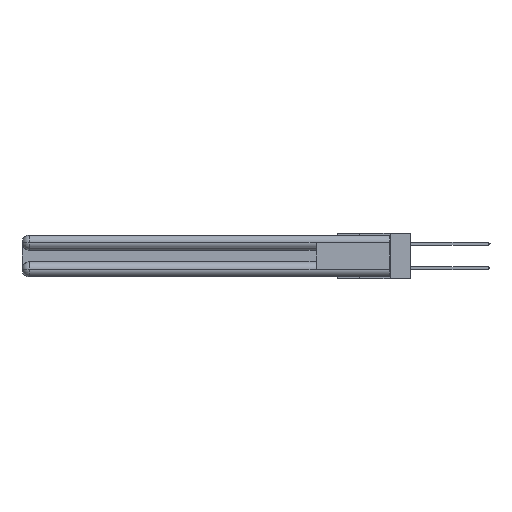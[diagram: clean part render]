
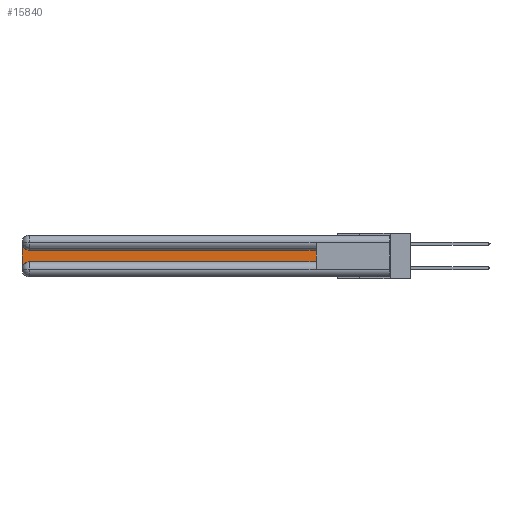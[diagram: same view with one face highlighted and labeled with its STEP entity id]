
A CAD part, left-side view. The second image highlights one B-rep face of the part: STEP entity #15840.
In plain terms, the highlighted planar face has unit normal (-1, 0, 0).
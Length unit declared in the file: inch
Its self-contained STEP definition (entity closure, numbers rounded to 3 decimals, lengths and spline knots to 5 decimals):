
#401 = VERTEX_POINT ( 'NONE', #23673 ) ;
#842 = DIRECTION ( 'NONE',  ( 0., -1., 0. ) ) ;
#939 = VERTEX_POINT ( 'NONE', #5828 ) ;
#1299 = CARTESIAN_POINT ( 'NONE',  ( 0.075, 0.6, -0.2175 ) ) ;
#1949 = EDGE_CURVE ( 'NONE', #9593, #939, #20219, .T. ) ;
#2138 = CARTESIAN_POINT ( 'NONE',  ( 0.075, 3., -0.2775 ) ) ;
#4886 = ORIENTED_EDGE ( 'NONE', *, *, #18905, .T. ) ;
#5600 = DIRECTION ( 'NONE',  ( 0., 1., 0. ) ) ;
#5828 = CARTESIAN_POINT ( 'NONE',  ( 0.075, 2.94, -0.2175 ) ) ;
#6166 = EDGE_LOOP ( 'NONE', ( #17412, #31448, #7244, #15046, #4886, #8875 ) ) ;
#6314 = VECTOR ( 'NONE', #21646, 39.37008 ) ;
#7009 = VECTOR ( 'NONE', #30650, 39.37008 ) ;
#7244 = ORIENTED_EDGE ( 'NONE', *, *, #7268, .T. ) ;
#7268 = EDGE_CURVE ( 'NONE', #401, #9593, #13897, .T. ) ;
#8222 = CARTESIAN_POINT ( 'NONE',  ( 0.075, 3., -0.1225 ) ) ;
#8849 = LINE ( 'NONE', #20236, #29769 ) ;
#8875 = ORIENTED_EDGE ( 'NONE', *, *, #17406, .T. ) ;
#9230 = VECTOR ( 'NONE', #842, 39.37008 ) ;
#9508 = DIRECTION ( 'NONE',  ( 0., 0., -1. ) ) ;
#9593 = VERTEX_POINT ( 'NONE', #2138 ) ;
#9915 = EDGE_CURVE ( 'NONE', #18895, #13813, #8849, .T. ) ;
#12706 = CARTESIAN_POINT ( 'NONE',  ( 0.075, 0.6, -0.2175 ) ) ;
#13439 = LINE ( 'NONE', #1299, #7009 ) ;
#13813 = VERTEX_POINT ( 'NONE', #14164 ) ;
#13897 = LINE ( 'NONE', #16421, #6314 ) ;
#14044 = CARTESIAN_POINT ( 'NONE',  ( 0.075, 0.6, -0.2175 ) ) ;
#14164 = CARTESIAN_POINT ( 'NONE',  ( 0.075, 2.94, -0.1225 ) ) ;
#15046 = ORIENTED_EDGE ( 'NONE', *, *, #1949, .T. ) ;
#15840 = ADVANCED_FACE ( 'NONE', ( #29545 ), #22667, .F. ) ;
#16421 = CARTESIAN_POINT ( 'NONE',  ( 0.075, 3., -0.2175 ) ) ;
#17406 = EDGE_CURVE ( 'NONE', #29827, #18895, #13439, .T. ) ;
#17412 = ORIENTED_EDGE ( 'NONE', *, *, #9915, .T. ) ;
#17721 = CARTESIAN_POINT ( 'NONE',  ( 0.075, 0.6, -0.1225 ) ) ;
#18531 = AXIS2_PLACEMENT_3D ( 'NONE', #25377, #23045, #30403 ) ;
#18895 = VERTEX_POINT ( 'NONE', #17721 ) ;
#18905 = EDGE_CURVE ( 'NONE', #939, #29827, #19487, .T. ) ;
#19487 = LINE ( 'NONE', #12706, #9230 ) ;
#19723 = AXIS2_PLACEMENT_3D ( 'NONE', #21421, #29066, #9508 ) ;
#20219 = CIRCLE ( 'NONE', #18531, 0.06 ) ;
#20236 = CARTESIAN_POINT ( 'NONE',  ( 0.075, 0.6, -0.1225 ) ) ;
#21421 = CARTESIAN_POINT ( 'NONE',  ( 0.075, 2.94, -0.0625 ) ) ;
#21646 = DIRECTION ( 'NONE',  ( 0., 0., -1. ) ) ;
#22275 = CIRCLE ( 'NONE', #19723, 0.06 ) ;
#22667 = PLANE ( 'NONE',  #26305 ) ;
#23045 = DIRECTION ( 'NONE',  ( 1., 0., 0. ) ) ;
#23673 = CARTESIAN_POINT ( 'NONE',  ( 0.075, 3., -0.0625 ) ) ;
#24008 = EDGE_CURVE ( 'NONE', #13813, #401, #22275, .T. ) ;
#25201 = DIRECTION ( 'NONE',  ( 1., 0., 0. ) ) ;
#25377 = CARTESIAN_POINT ( 'NONE',  ( 0.075, 2.94, -0.2775 ) ) ;
#26305 = AXIS2_PLACEMENT_3D ( 'NONE', #8222, #25201, #30121 ) ;
#29066 = DIRECTION ( 'NONE',  ( 1., 0., 0. ) ) ;
#29545 = FACE_OUTER_BOUND ( 'NONE', #6166, .T. ) ;
#29769 = VECTOR ( 'NONE', #5600, 39.37008 ) ;
#29827 = VERTEX_POINT ( 'NONE', #14044 ) ;
#30121 = DIRECTION ( 'NONE',  ( 0., 0., -1. ) ) ;
#30403 = DIRECTION ( 'NONE',  ( 0., 0., -1. ) ) ;
#30650 = DIRECTION ( 'NONE',  ( 0., 0., 1. ) ) ;
#31448 = ORIENTED_EDGE ( 'NONE', *, *, #24008, .T. ) ;
